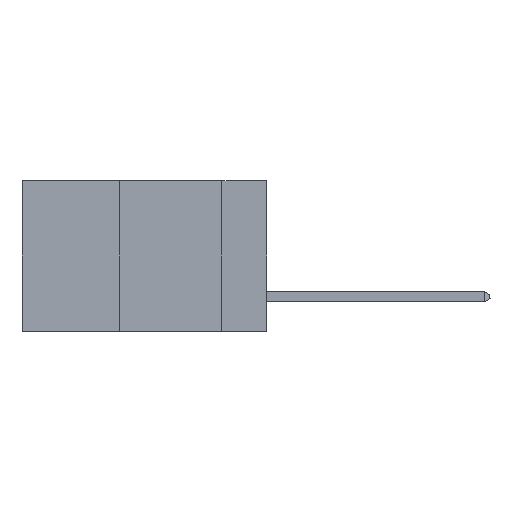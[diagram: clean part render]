
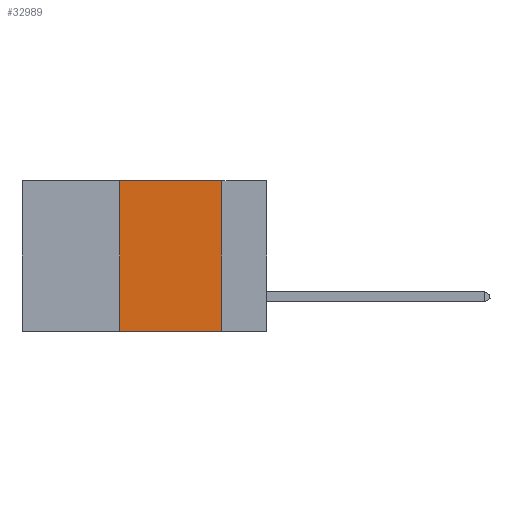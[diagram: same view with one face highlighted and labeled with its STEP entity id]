
A CAD part, left-side view. The second image highlights one B-rep face of the part: STEP entity #32989.
In plain terms, the highlighted planar face has unit normal (-1, 0, 0).
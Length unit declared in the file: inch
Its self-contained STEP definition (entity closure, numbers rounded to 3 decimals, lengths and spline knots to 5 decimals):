
#460 = EDGE_CURVE ( 'NONE', #35267, #13298, #16147, .T. ) ;
#845 = LINE ( 'NONE', #37149, #28310 ) ;
#4981 = VECTOR ( 'NONE', #26574, 39.37008 ) ;
#6604 = CARTESIAN_POINT ( 'NONE',  ( 0., 0.36, 0. ) ) ;
#7455 = ORIENTED_EDGE ( 'NONE', *, *, #28135, .F. ) ;
#9563 = LINE ( 'NONE', #19926, #4981 ) ;
#9776 = DIRECTION ( 'NONE',  ( 0., 0., 1. ) ) ;
#12009 = LINE ( 'NONE', #19491, #20170 ) ;
#12321 = CARTESIAN_POINT ( 'NONE',  ( 0., 0.6, -0.37 ) ) ;
#13287 = EDGE_CURVE ( 'NONE', #35267, #27549, #12009, .T. ) ;
#13298 = VERTEX_POINT ( 'NONE', #29146 ) ;
#13358 = VERTEX_POINT ( 'NONE', #16286 ) ;
#14748 = DIRECTION ( 'NONE',  ( 0., -1., 0. ) ) ;
#16147 = LINE ( 'NONE', #12321, #19685 ) ;
#16286 = CARTESIAN_POINT ( 'NONE',  ( 0., 0.11, 0. ) ) ;
#18373 = PLANE ( 'NONE',  #34212 ) ;
#19491 = CARTESIAN_POINT ( 'NONE',  ( 0., 0.36, 0. ) ) ;
#19685 = VECTOR ( 'NONE', #28254, 39.37008 ) ;
#19926 = CARTESIAN_POINT ( 'NONE',  ( 0., 0.11, 0. ) ) ;
#20170 = VECTOR ( 'NONE', #9776, 39.37008 ) ;
#25030 = CARTESIAN_POINT ( 'NONE',  ( 0., 0.6, 0. ) ) ;
#25269 = CARTESIAN_POINT ( 'NONE',  ( 0., 0.36, -0.37 ) ) ;
#25655 = EDGE_LOOP ( 'NONE', ( #7455, #26615, #40170, #41870 ) ) ;
#26574 = DIRECTION ( 'NONE',  ( 0., 0., -1. ) ) ;
#26615 = ORIENTED_EDGE ( 'NONE', *, *, #31774, .F. ) ;
#27549 = VERTEX_POINT ( 'NONE', #6604 ) ;
#28135 = EDGE_CURVE ( 'NONE', #13358, #13298, #9563, .T. ) ;
#28254 = DIRECTION ( 'NONE',  ( 0., -1., 0. ) ) ;
#28310 = VECTOR ( 'NONE', #14748, 39.37008 ) ;
#29146 = CARTESIAN_POINT ( 'NONE',  ( 0., 0.11, -0.37 ) ) ;
#31433 = DIRECTION ( 'NONE',  ( 0., 0., -1. ) ) ;
#31774 = EDGE_CURVE ( 'NONE', #27549, #13358, #845, .T. ) ;
#32989 = ADVANCED_FACE ( 'NONE', ( #38955 ), #18373, .F. ) ;
#34212 = AXIS2_PLACEMENT_3D ( 'NONE', #25030, #40958, #31433 ) ;
#35267 = VERTEX_POINT ( 'NONE', #25269 ) ;
#37149 = CARTESIAN_POINT ( 'NONE',  ( 0., 0.6, 0. ) ) ;
#38955 = FACE_OUTER_BOUND ( 'NONE', #25655, .T. ) ;
#40170 = ORIENTED_EDGE ( 'NONE', *, *, #13287, .F. ) ;
#40958 = DIRECTION ( 'NONE',  ( 1., 0., 0. ) ) ;
#41870 = ORIENTED_EDGE ( 'NONE', *, *, #460, .T. ) ;
